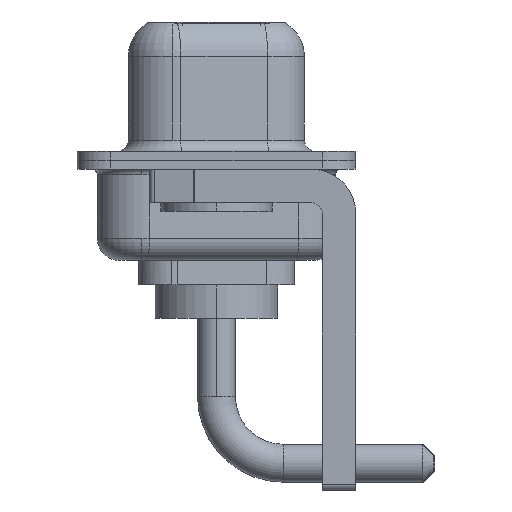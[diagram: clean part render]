
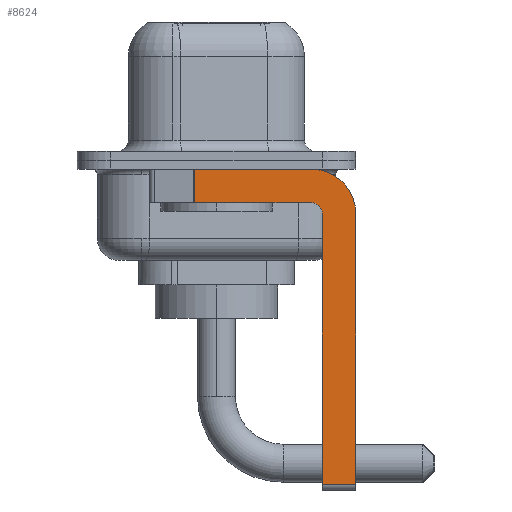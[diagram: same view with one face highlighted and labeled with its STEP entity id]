
A CAD part, left-side view. The second image highlights one B-rep face of the part: STEP entity #8624.
In plain terms, the highlighted planar face has unit normal (-1, 0, 0).
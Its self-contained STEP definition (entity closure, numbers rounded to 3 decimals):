
#367 = VECTOR ( 'NONE', #1939, 1000. ) ;
#373 = DIRECTION ( 'NONE',  ( 0., -1., 0. ) ) ;
#474 = VERTEX_POINT ( 'NONE', #1169 ) ;
#605 = AXIS2_PLACEMENT_3D ( 'NONE', #3202, #13302, #11370 ) ;
#685 = VERTEX_POINT ( 'NONE', #9569 ) ;
#868 = AXIS2_PLACEMENT_3D ( 'NONE', #3712, #8200, #11448 ) ;
#1169 = CARTESIAN_POINT ( 'NONE',  ( -2.9, -6.25, -2.4 ) ) ;
#1205 = LINE ( 'NONE', #3197, #1740 ) ;
#1380 = ORIENTED_EDGE ( 'NONE', *, *, #2475, .F. ) ;
#1617 = CARTESIAN_POINT ( 'NONE',  ( -2.9, -4.25, -14.55 ) ) ;
#1688 = VECTOR ( 'NONE', #2880, 1000. ) ;
#1740 = VECTOR ( 'NONE', #6579, 1000. ) ;
#1936 = EDGE_CURVE ( 'NONE', #685, #2527, #9425, .T. ) ;
#1939 = DIRECTION ( 'NONE',  ( 0., -1., 0. ) ) ;
#2098 = VERTEX_POINT ( 'NONE', #14294 ) ;
#2475 = EDGE_CURVE ( 'NONE', #11433, #13025, #3051, .T. ) ;
#2527 = VERTEX_POINT ( 'NONE', #14059 ) ;
#2843 = ORIENTED_EDGE ( 'NONE', *, *, #1936, .F. ) ;
#2851 = CARTESIAN_POINT ( 'NONE',  ( -2.9, -4.75, -14.8 ) ) ;
#2880 = DIRECTION ( 'NONE',  ( 0., 0., -1. ) ) ;
#2881 = DIRECTION ( 'NONE',  ( 0., 0., -1. ) ) ;
#2933 = EDGE_CURVE ( 'NONE', #13025, #474, #8833, .T. ) ;
#3051 = LINE ( 'NONE', #5189, #367 ) ;
#3197 = CARTESIAN_POINT ( 'NONE',  ( -2.9, -6.25, -2.4 ) ) ;
#3202 = CARTESIAN_POINT ( 'NONE',  ( -2.9, -4.25, -2.4 ) ) ;
#3712 = CARTESIAN_POINT ( 'NONE',  ( -2.9, -4.25, -2.4 ) ) ;
#3768 = ORIENTED_EDGE ( 'NONE', *, *, #10589, .F. ) ;
#3937 = ORIENTED_EDGE ( 'NONE', *, *, #2933, .F. ) ;
#3965 = DIRECTION ( 'NONE',  ( 0., 0., 1. ) ) ;
#5189 = CARTESIAN_POINT ( 'NONE',  ( -2.9, 3., -0.4 ) ) ;
#5942 = LINE ( 'NONE', #1617, #7286 ) ;
#6191 = CARTESIAN_POINT ( 'NONE',  ( -2.9, 0.978, -1.9 ) ) ;
#6280 = CARTESIAN_POINT ( 'NONE',  ( -2.9, -4.25, -2.4 ) ) ;
#6579 = DIRECTION ( 'NONE',  ( 0., 0., -1. ) ) ;
#6924 = ORIENTED_EDGE ( 'NONE', *, *, #10218, .T. ) ;
#6947 = FACE_OUTER_BOUND ( 'NONE', #9142, .T. ) ;
#7286 = VECTOR ( 'NONE', #373, 1000. ) ;
#7738 = ORIENTED_EDGE ( 'NONE', *, *, #9316, .F. ) ;
#8025 = CARTESIAN_POINT ( 'NONE',  ( -2.9, 0.978, -1.9 ) ) ;
#8200 = DIRECTION ( 'NONE',  ( 1., 0., 0. ) ) ;
#8624 = ADVANCED_FACE ( 'NONE', ( #6947 ), #11598, .F. ) ;
#8833 = CIRCLE ( 'NONE', #9781, 2. ) ;
#8970 = EDGE_CURVE ( 'NONE', #685, #13381, #5942, .T. ) ;
#9142 = EDGE_LOOP ( 'NONE', ( #1380, #6924, #7738, #10374, #2843, #10789, #3768, #3937 ) ) ;
#9316 = EDGE_CURVE ( 'NONE', #2098, #13977, #13390, .T. ) ;
#9425 = LINE ( 'NONE', #2851, #10699 ) ;
#9569 = CARTESIAN_POINT ( 'NONE',  ( -2.9, -4.75, -14.55 ) ) ;
#9740 = DIRECTION ( 'NONE',  ( 1., 0., 0. ) ) ;
#9781 = AXIS2_PLACEMENT_3D ( 'NONE', #6280, #9740, #2881 ) ;
#10218 = EDGE_CURVE ( 'NONE', #11433, #13977, #10485, .T. ) ;
#10374 = ORIENTED_EDGE ( 'NONE', *, *, #11963, .F. ) ;
#10485 = LINE ( 'NONE', #6191, #1688 ) ;
#10589 = EDGE_CURVE ( 'NONE', #474, #13381, #1205, .T. ) ;
#10699 = VECTOR ( 'NONE', #3965, 1000. ) ;
#10789 = ORIENTED_EDGE ( 'NONE', *, *, #8970, .T. ) ;
#10916 = VECTOR ( 'NONE', #12491, 1000. ) ;
#11207 = CARTESIAN_POINT ( 'NONE',  ( -2.9, -4.25, -0.4 ) ) ;
#11370 = DIRECTION ( 'NONE',  ( 0., 0., 1. ) ) ;
#11433 = VERTEX_POINT ( 'NONE', #14220 ) ;
#11448 = DIRECTION ( 'NONE',  ( 0., 0., -1. ) ) ;
#11469 = CARTESIAN_POINT ( 'NONE',  ( -2.9, -4.25, -1.9 ) ) ;
#11598 = PLANE ( 'NONE',  #868 ) ;
#11963 = EDGE_CURVE ( 'NONE', #2527, #2098, #12350, .T. ) ;
#12350 = CIRCLE ( 'NONE', #605, 0.5 ) ;
#12491 = DIRECTION ( 'NONE',  ( 0., 1., 0. ) ) ;
#13025 = VERTEX_POINT ( 'NONE', #11207 ) ;
#13121 = CARTESIAN_POINT ( 'NONE',  ( -2.9, -6.25, -14.55 ) ) ;
#13302 = DIRECTION ( 'NONE',  ( -1., 0., 0. ) ) ;
#13381 = VERTEX_POINT ( 'NONE', #13121 ) ;
#13390 = LINE ( 'NONE', #11469, #10916 ) ;
#13977 = VERTEX_POINT ( 'NONE', #8025 ) ;
#14059 = CARTESIAN_POINT ( 'NONE',  ( -2.9, -4.75, -2.4 ) ) ;
#14220 = CARTESIAN_POINT ( 'NONE',  ( -2.9, 0.978, -0.4 ) ) ;
#14294 = CARTESIAN_POINT ( 'NONE',  ( -2.9, -4.25, -1.9 ) ) ;
